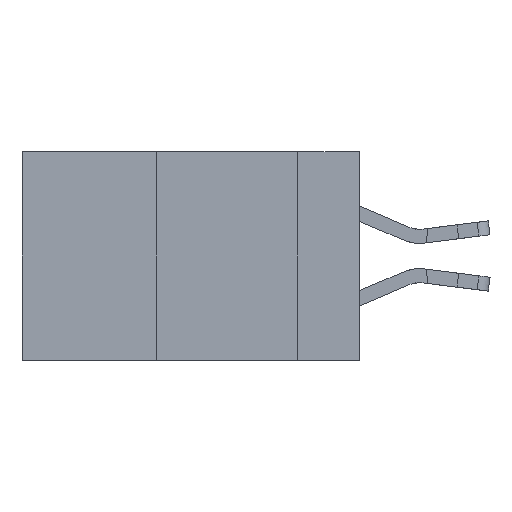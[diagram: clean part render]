
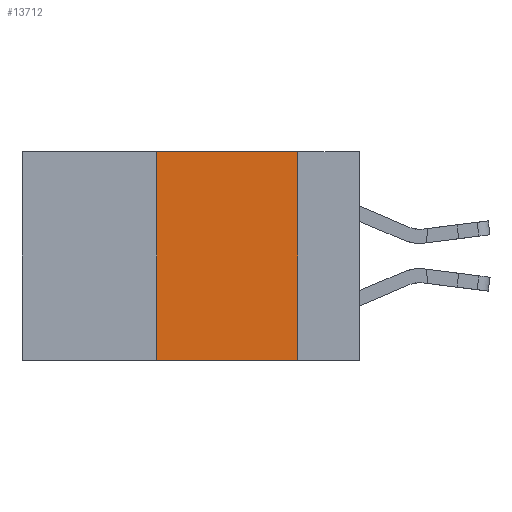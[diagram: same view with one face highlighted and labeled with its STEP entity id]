
A CAD part, left-side view. The second image highlights one B-rep face of the part: STEP entity #13712.
In plain terms, the highlighted planar face has unit normal (-1, 0, 0).
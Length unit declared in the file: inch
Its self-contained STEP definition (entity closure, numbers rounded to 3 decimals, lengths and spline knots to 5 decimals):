
#17 = ORIENTED_EDGE ( 'NONE', *, *, #179, .T. ) ;
#179 = EDGE_CURVE ( 'NONE', #11855, #2274, #14846, .T. ) ;
#1470 = LINE ( 'NONE', #2017, #6154 ) ;
#1558 = DIRECTION ( 'NONE',  ( 0., 0., -1. ) ) ;
#1701 = LINE ( 'NONE', #3849, #16409 ) ;
#1764 = DIRECTION ( 'NONE',  ( 1., 0., 0. ) ) ;
#2017 = CARTESIAN_POINT ( 'NONE',  ( 0., 0.36, 0. ) ) ;
#2039 = VERTEX_POINT ( 'NONE', #2810 ) ;
#2092 = CARTESIAN_POINT ( 'NONE',  ( 0., 0.6, -0.37 ) ) ;
#2274 = VERTEX_POINT ( 'NONE', #2858 ) ;
#2275 = DIRECTION ( 'NONE',  ( 0., -1., 0. ) ) ;
#2810 = CARTESIAN_POINT ( 'NONE',  ( 0., 0.11, 0. ) ) ;
#2858 = CARTESIAN_POINT ( 'NONE',  ( 0., 0.11, -0.37 ) ) ;
#3849 = CARTESIAN_POINT ( 'NONE',  ( 0., 0.11, 0. ) ) ;
#4057 = EDGE_CURVE ( 'NONE', #11855, #8549, #1470, .T. ) ;
#4404 = CARTESIAN_POINT ( 'NONE',  ( 0., 0.36, -0.37 ) ) ;
#4509 = CARTESIAN_POINT ( 'NONE',  ( 0., 0.6, 0. ) ) ;
#4645 = CARTESIAN_POINT ( 'NONE',  ( 0., 0.6, 0. ) ) ;
#5892 = EDGE_CURVE ( 'NONE', #8549, #2039, #9975, .T. ) ;
#6154 = VECTOR ( 'NONE', #19485, 39.37008 ) ;
#6770 = ORIENTED_EDGE ( 'NONE', *, *, #5892, .F. ) ;
#8492 = VECTOR ( 'NONE', #18695, 39.37008 ) ;
#8549 = VERTEX_POINT ( 'NONE', #12760 ) ;
#9113 = ORIENTED_EDGE ( 'NONE', *, *, #18362, .F. ) ;
#9975 = LINE ( 'NONE', #4509, #8492 ) ;
#10887 = AXIS2_PLACEMENT_3D ( 'NONE', #4645, #1764, #1558 ) ;
#11082 = PLANE ( 'NONE',  #10887 ) ;
#11437 = VECTOR ( 'NONE', #2275, 39.37008 ) ;
#11855 = VERTEX_POINT ( 'NONE', #4404 ) ;
#11964 = FACE_OUTER_BOUND ( 'NONE', #15734, .T. ) ;
#12760 = CARTESIAN_POINT ( 'NONE',  ( 0., 0.36, 0. ) ) ;
#12868 = ORIENTED_EDGE ( 'NONE', *, *, #4057, .F. ) ;
#13712 = ADVANCED_FACE ( 'NONE', ( #11964 ), #11082, .F. ) ;
#14846 = LINE ( 'NONE', #2092, #11437 ) ;
#15734 = EDGE_LOOP ( 'NONE', ( #9113, #6770, #12868, #17 ) ) ;
#16409 = VECTOR ( 'NONE', #19102, 39.37008 ) ;
#18362 = EDGE_CURVE ( 'NONE', #2039, #2274, #1701, .T. ) ;
#18695 = DIRECTION ( 'NONE',  ( 0., -1., 0. ) ) ;
#19102 = DIRECTION ( 'NONE',  ( 0., 0., -1. ) ) ;
#19485 = DIRECTION ( 'NONE',  ( 0., 0., 1. ) ) ;
